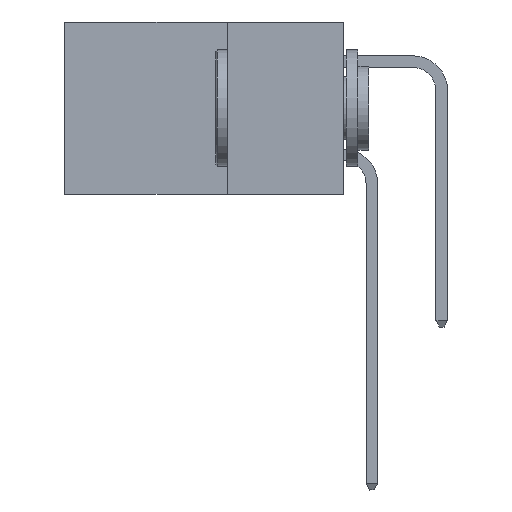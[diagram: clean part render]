
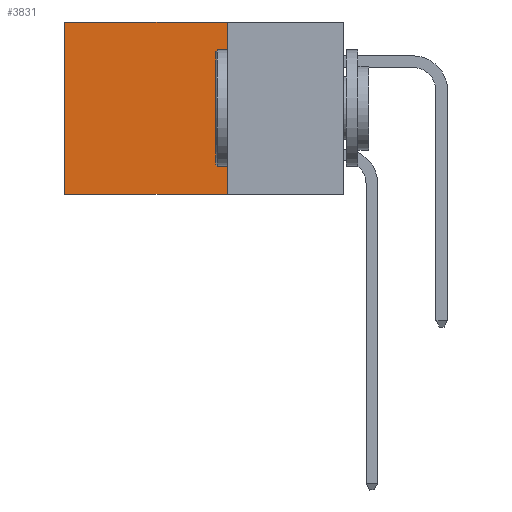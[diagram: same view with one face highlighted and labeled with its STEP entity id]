
A CAD part, left-side view. The second image highlights one B-rep face of the part: STEP entity #3831.
In plain terms, the highlighted planar face has unit normal (-1, 0, 0).
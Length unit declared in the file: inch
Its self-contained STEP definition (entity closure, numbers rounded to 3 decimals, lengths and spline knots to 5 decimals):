
#2528 = CARTESIAN_POINT ( 'NONE',  ( 0.2615, 0.25, -0.37 ) ) ;
#3831 = ADVANCED_FACE ( 'NONE', ( #20427 ), #19399, .F. ) ;
#4504 = CARTESIAN_POINT ( 'NONE',  ( 0.2615, 0.25, -0.37 ) ) ;
#4537 = LINE ( 'NONE', #24302, #26893 ) ;
#4873 = ORIENTED_EDGE ( 'NONE', *, *, #9945, .F. ) ;
#5309 = VERTEX_POINT ( 'NONE', #25898 ) ;
#5827 = ORIENTED_EDGE ( 'NONE', *, *, #23109, .T. ) ;
#5992 = DIRECTION ( 'NONE',  ( 0., 0., -1. ) ) ;
#6245 = LINE ( 'NONE', #4504, #12959 ) ;
#7003 = VERTEX_POINT ( 'NONE', #16317 ) ;
#7112 = VECTOR ( 'NONE', #5992, 39.37008 ) ;
#7704 = EDGE_CURVE ( 'NONE', #16573, #5309, #12417, .T. ) ;
#8071 = VERTEX_POINT ( 'NONE', #11632 ) ;
#8850 = ORIENTED_EDGE ( 'NONE', *, *, #7704, .F. ) ;
#9069 = DIRECTION ( 'NONE',  ( 0., 1., 0. ) ) ;
#9945 = EDGE_CURVE ( 'NONE', #5309, #8071, #6245, .T. ) ;
#11610 = VECTOR ( 'NONE', #24800, 39.37008 ) ;
#11632 = CARTESIAN_POINT ( 'NONE',  ( 0.2615, 0.6, -0.37 ) ) ;
#12417 = LINE ( 'NONE', #19433, #7112 ) ;
#12959 = VECTOR ( 'NONE', #9069, 39.37008 ) ;
#13350 = EDGE_CURVE ( 'NONE', #16573, #7003, #4537, .T. ) ;
#15101 = ORIENTED_EDGE ( 'NONE', *, *, #13350, .T. ) ;
#16317 = CARTESIAN_POINT ( 'NONE',  ( 0.2615, 0.6, 0. ) ) ;
#16573 = VERTEX_POINT ( 'NONE', #20181 ) ;
#19399 = PLANE ( 'NONE',  #19944 ) ;
#19433 = CARTESIAN_POINT ( 'NONE',  ( 0.2615, 0.25, -0.37 ) ) ;
#19933 = DIRECTION ( 'NONE',  ( 0., 1., 0. ) ) ;
#19944 = AXIS2_PLACEMENT_3D ( 'NONE', #2528, #22926, #22997 ) ;
#20181 = CARTESIAN_POINT ( 'NONE',  ( 0.2615, 0.25, 0. ) ) ;
#20427 = FACE_OUTER_BOUND ( 'NONE', #24876, .T. ) ;
#22569 = CARTESIAN_POINT ( 'NONE',  ( 0.2615, 0.6, -0.37 ) ) ;
#22926 = DIRECTION ( 'NONE',  ( 1., 0., 0. ) ) ;
#22997 = DIRECTION ( 'NONE',  ( 0., 0., -1. ) ) ;
#23109 = EDGE_CURVE ( 'NONE', #7003, #8071, #23457, .T. ) ;
#23457 = LINE ( 'NONE', #22569, #11610 ) ;
#24302 = CARTESIAN_POINT ( 'NONE',  ( 0.2615, 0.25, 0. ) ) ;
#24800 = DIRECTION ( 'NONE',  ( 0., 0., -1. ) ) ;
#24876 = EDGE_LOOP ( 'NONE', ( #5827, #4873, #8850, #15101 ) ) ;
#25898 = CARTESIAN_POINT ( 'NONE',  ( 0.2615, 0.25, -0.37 ) ) ;
#26893 = VECTOR ( 'NONE', #19933, 39.37008 ) ;
